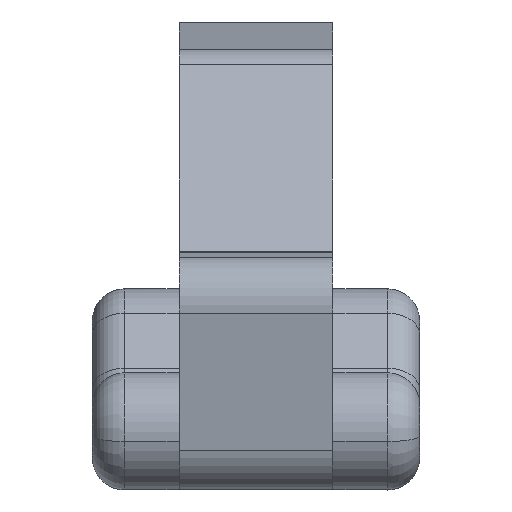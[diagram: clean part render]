
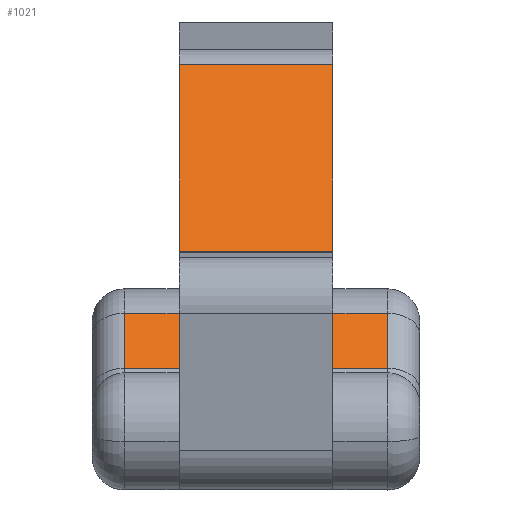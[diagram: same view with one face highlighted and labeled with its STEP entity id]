
A CAD part, left-side view. The second image highlights one B-rep face of the part: STEP entity #1021.
In plain terms, the highlighted planar face has unit normal (-0.745, 0, 0.667).
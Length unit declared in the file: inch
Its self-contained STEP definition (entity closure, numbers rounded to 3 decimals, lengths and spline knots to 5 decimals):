
#3 = CARTESIAN_POINT ( 'NONE',  ( 0.47849, -0.36657, 0.01919 ) ) ;
#15 = DIRECTION ( 'NONE',  ( 0., 1., 0. ) ) ;
#37 = CARTESIAN_POINT ( 'NONE',  ( 0.47849, -0.36657, 0.01919 ) ) ;
#48 = VECTOR ( 'NONE', #291, 39.37008 ) ;
#54 = VECTOR ( 'NONE', #427, 39.37008 ) ;
#95 = VERTEX_POINT ( 'NONE', #1198 ) ;
#127 = EDGE_CURVE ( 'NONE', #363, #140, #271, .T. ) ;
#140 = VERTEX_POINT ( 'NONE', #532 ) ;
#147 = DIRECTION ( 'NONE',  ( 0., 1., 0. ) ) ;
#159 = EDGE_CURVE ( 'NONE', #1575, #1425, #557, .T. ) ;
#162 = CARTESIAN_POINT ( 'NONE',  ( 0.47849, -0.23107, 0.01919 ) ) ;
#176 = EDGE_CURVE ( 'NONE', #617, #1575, #1082, .T. ) ;
#202 = CARTESIAN_POINT ( 'NONE',  ( 0.47849, 0.09443, 0.01919 ) ) ;
#230 = FACE_OUTER_BOUND ( 'NONE', #604, .T. ) ;
#261 = EDGE_CURVE ( 'NONE', #95, #617, #1112, .T. ) ;
#271 = LINE ( 'NONE', #1628, #950 ) ;
#291 = DIRECTION ( 'NONE',  ( -0.667, 0., -0.745 ) ) ;
#315 = AXIS2_PLACEMENT_3D ( 'NONE', #1372, #1673, #1240 ) ;
#316 = EDGE_CURVE ( 'NONE', #363, #1755, #522, .T. ) ;
#356 = ORIENTED_EDGE ( 'NONE', *, *, #316, .T. ) ;
#363 = VERTEX_POINT ( 'NONE', #1697 ) ;
#373 = ORIENTED_EDGE ( 'NONE', *, *, #1176, .T. ) ;
#427 = DIRECTION ( 'NONE',  ( 0., 1., 0. ) ) ;
#464 = EDGE_CURVE ( 'NONE', #95, #1217, #1572, .T. ) ;
#475 = VECTOR ( 'NONE', #15, 39.37008 ) ;
#522 = LINE ( 'NONE', #1400, #651 ) ;
#528 = LINE ( 'NONE', #37, #54 ) ;
#532 = CARTESIAN_POINT ( 'NONE',  ( 0.40157, 0.09443, -0.06675 ) ) ;
#554 = CARTESIAN_POINT ( 'NONE',  ( 0.82573, -0.23107, 0.40716 ) ) ;
#557 = LINE ( 'NONE', #3, #475 ) ;
#604 = EDGE_LOOP ( 'NONE', ( #812, #373, #1622, #356, #938, #1727, #738, #1486 ) ) ;
#617 = VERTEX_POINT ( 'NONE', #629 ) ;
#629 = CARTESIAN_POINT ( 'NONE',  ( 0.82573, 0.00893, 0.40716 ) ) ;
#651 = VECTOR ( 'NONE', #1387, 39.37008 ) ;
#738 = ORIENTED_EDGE ( 'NONE', *, *, #261, .T. ) ;
#812 = ORIENTED_EDGE ( 'NONE', *, *, #159, .T. ) ;
#813 = PLANE ( 'NONE',  #315 ) ;
#814 = CARTESIAN_POINT ( 'NONE',  ( 0.47849, -0.31657, 0.01919 ) ) ;
#823 = VECTOR ( 'NONE', #1556, 39.37008 ) ;
#849 = CARTESIAN_POINT ( 'NONE',  ( 0.40157, 0.09443, -0.06675 ) ) ;
#882 = CARTESIAN_POINT ( 'NONE',  ( 0.47849, 0.00893, 0.01919 ) ) ;
#884 = VECTOR ( 'NONE', #954, 39.37008 ) ;
#938 = ORIENTED_EDGE ( 'NONE', *, *, #1062, .T. ) ;
#950 = VECTOR ( 'NONE', #147, 39.37008 ) ;
#954 = DIRECTION ( 'NONE',  ( 0., 1., 0. ) ) ;
#994 = CARTESIAN_POINT ( 'NONE',  ( 0.40157, -0.23107, -0.06675 ) ) ;
#1021 = ADVANCED_FACE ( 'NONE', ( #230 ), #813, .F. ) ;
#1062 = EDGE_CURVE ( 'NONE', #1755, #1217, #528, .T. ) ;
#1082 = LINE ( 'NONE', #1506, #48 ) ;
#1112 = LINE ( 'NONE', #554, #884 ) ;
#1116 = DIRECTION ( 'NONE',  ( -0.667, 0., -0.745 ) ) ;
#1176 = EDGE_CURVE ( 'NONE', #1425, #140, #1287, .T. ) ;
#1198 = CARTESIAN_POINT ( 'NONE',  ( 0.82573, -0.23107, 0.40716 ) ) ;
#1217 = VERTEX_POINT ( 'NONE', #162 ) ;
#1240 = DIRECTION ( 'NONE',  ( 0.667, 0., 0.745 ) ) ;
#1287 = LINE ( 'NONE', #849, #1449 ) ;
#1372 = CARTESIAN_POINT ( 'NONE',  ( 0.40157, -0.23107, -0.06675 ) ) ;
#1387 = DIRECTION ( 'NONE',  ( 0.667, 0., 0.745 ) ) ;
#1400 = CARTESIAN_POINT ( 'NONE',  ( 0.47849, -0.31657, 0.01919 ) ) ;
#1425 = VERTEX_POINT ( 'NONE', #202 ) ;
#1449 = VECTOR ( 'NONE', #1116, 39.37008 ) ;
#1486 = ORIENTED_EDGE ( 'NONE', *, *, #176, .T. ) ;
#1506 = CARTESIAN_POINT ( 'NONE',  ( 0.40157, 0.00893, -0.06675 ) ) ;
#1556 = DIRECTION ( 'NONE',  ( -0.667, 0., -0.745 ) ) ;
#1572 = LINE ( 'NONE', #994, #823 ) ;
#1575 = VERTEX_POINT ( 'NONE', #882 ) ;
#1622 = ORIENTED_EDGE ( 'NONE', *, *, #127, .F. ) ;
#1628 = CARTESIAN_POINT ( 'NONE',  ( 0.40157, -0.23107, -0.06675 ) ) ;
#1673 = DIRECTION ( 'NONE',  ( 0.745, 0., -0.667 ) ) ;
#1697 = CARTESIAN_POINT ( 'NONE',  ( 0.40157, -0.31657, -0.06675 ) ) ;
#1727 = ORIENTED_EDGE ( 'NONE', *, *, #464, .F. ) ;
#1755 = VERTEX_POINT ( 'NONE', #814 ) ;
